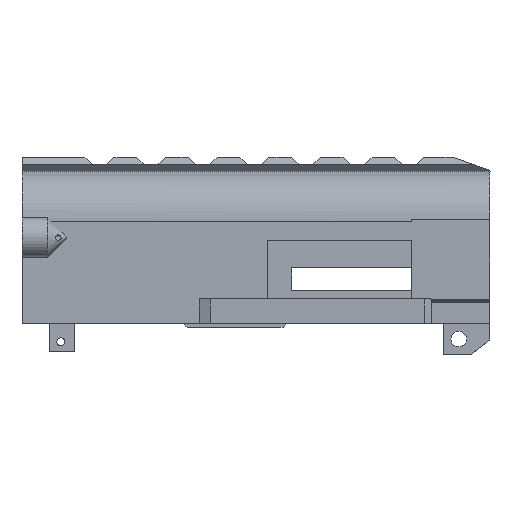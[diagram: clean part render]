
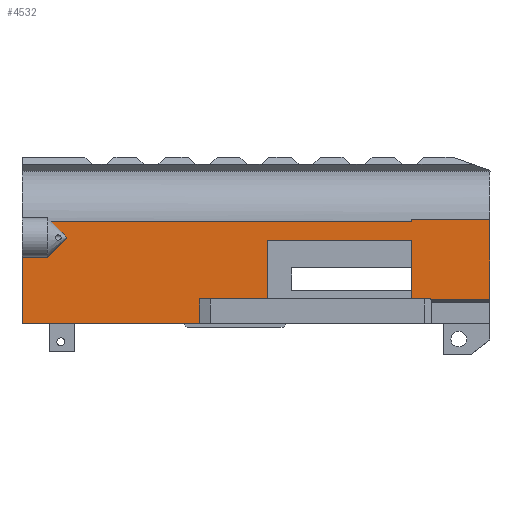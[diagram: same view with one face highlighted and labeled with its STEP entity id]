
A CAD part, top view. The second image highlights one B-rep face of the part: STEP entity #4532.
In plain terms, the highlighted planar face has unit normal (0, 0, 1).
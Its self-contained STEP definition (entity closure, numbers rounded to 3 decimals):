
#65 = CARTESIAN_POINT ( 'NONE',  ( -19.05, 16.229, 20.1 ) ) ;
#80 = VERTEX_POINT ( 'NONE', #4451 ) ;
#230 = CARTESIAN_POINT ( 'NONE',  ( -53.554, 16.363, 20.1 ) ) ;
#297 = DIRECTION ( 'NONE',  ( -1., 0., 0. ) ) ;
#432 = CARTESIAN_POINT ( 'NONE',  ( -11.605, 5.648, 20.1 ) ) ;
#480 = ORIENTED_EDGE ( 'NONE', *, *, #613, .F. ) ;
#537 = CARTESIAN_POINT ( 'NONE',  ( -167.482, 33.3, 20.1 ) ) ;
#572 = DIRECTION ( 'NONE',  ( 0.707, -0.707, 0. ) ) ;
#579 = VERTEX_POINT ( 'NONE', #3620 ) ;
#612 = LINE ( 'NONE', #2667, #9085 ) ;
#613 = EDGE_CURVE ( 'NONE', #3606, #579, #7584, .T. ) ;
#638 = DIRECTION ( 'NONE',  ( 1., 0., 0. ) ) ;
#674 = EDGE_LOOP ( 'NONE', ( #7659, #3589, #480, #2701, #2928, #7825, #6743, #4320, #2395, #4834, #3964, #5488, #8980, #8319, #5540, #8582, #5703, #3328 ) ) ;
#764 = VERTEX_POINT ( 'NONE', #1756 ) ;
#797 = EDGE_CURVE ( 'NONE', #6819, #8381, #4571, .T. ) ;
#798 = DIRECTION ( 'NONE',  ( -1., 0., 0. ) ) ;
#834 = AXIS2_PLACEMENT_3D ( 'NONE', #6555, #2433, #5251 ) ;
#867 = LINE ( 'NONE', #8546, #1990 ) ;
#907 = CARTESIAN_POINT ( 'NONE',  ( -177.682, 6.363, 20.1 ) ) ;
#932 = CARTESIAN_POINT ( 'NONE',  ( -78., 39.948, 20.1 ) ) ;
#972 = CARTESIAN_POINT ( 'NONE',  ( -159.682, 47.463, 20.1 ) ) ;
#995 = LINE ( 'NONE', #5081, #5765 ) ;
#1028 = VECTOR ( 'NONE', #638, 1000. ) ;
#1035 = DIRECTION ( 'NONE',  ( 0., -1., 0. ) ) ;
#1101 = VERTEX_POINT ( 'NONE', #8538 ) ;
#1129 = VECTOR ( 'NONE', #1190, 1000. ) ;
#1165 = LINE ( 'NONE', #7304, #7152 ) ;
#1190 = DIRECTION ( 'NONE',  ( -1., 0., 0. ) ) ;
#1319 = VERTEX_POINT ( 'NONE', #7970 ) ;
#1375 = CARTESIAN_POINT ( 'NONE',  ( -78., 16.363, 20.1 ) ) ;
#1378 = LINE ( 'NONE', #8827, #7618 ) ;
#1498 = CARTESIAN_POINT ( 'NONE',  ( -53.554, 16.363, 20.1 ) ) ;
#1505 = DIRECTION ( 'NONE',  ( 0., 1., 0. ) ) ;
#1574 = VECTOR ( 'NONE', #5190, 1000. ) ;
#1577 = DIRECTION ( 'NONE',  ( 1., 0., 0. ) ) ;
#1581 = VECTOR ( 'NONE', #1035, 1000. ) ;
#1756 = CARTESIAN_POINT ( 'NONE',  ( -11.605, 16.229, 20.1 ) ) ;
#1922 = CARTESIAN_POINT ( 'NONE',  ( -39.772, 39.948, 20.1 ) ) ;
#1963 = EDGE_CURVE ( 'NONE', #5956, #764, #5717, .T. ) ;
#1990 = VECTOR ( 'NONE', #1505, 1000. ) ;
#2395 = ORIENTED_EDGE ( 'NONE', *, *, #9096, .F. ) ;
#2433 = DIRECTION ( 'NONE',  ( 0., 0., 1. ) ) ;
#2667 = CARTESIAN_POINT ( 'NONE',  ( -159.482, 41.3, 20.1 ) ) ;
#2699 = LINE ( 'NONE', #972, #1581 ) ;
#2701 = ORIENTED_EDGE ( 'NONE', *, *, #6068, .T. ) ;
#2803 = VECTOR ( 'NONE', #6584, 1000. ) ;
#2820 = EDGE_CURVE ( 'NONE', #5543, #8736, #8386, .T. ) ;
#2871 = CARTESIAN_POINT ( 'NONE',  ( -105.565, 6.363, 20.1 ) ) ;
#2928 = ORIENTED_EDGE ( 'NONE', *, *, #7368, .F. ) ;
#3069 = CARTESIAN_POINT ( 'NONE',  ( -19.032, 39.948, 20.1 ) ) ;
#3086 = PLANE ( 'NONE',  #834 ) ;
#3224 = CARTESIAN_POINT ( 'NONE',  ( -159.682, 41.1, 20.1 ) ) ;
#3283 = LINE ( 'NONE', #4553, #7811 ) ;
#3308 = DIRECTION ( 'NONE',  ( 0., -1., 0. ) ) ;
#3311 = CARTESIAN_POINT ( 'NONE',  ( -43.5, 6.363, 20.1 ) ) ;
#3328 = ORIENTED_EDGE ( 'NONE', *, *, #6326, .T. ) ;
#3572 = LINE ( 'NONE', #4238, #7133 ) ;
#3589 = ORIENTED_EDGE ( 'NONE', *, *, #6388, .F. ) ;
#3606 = VERTEX_POINT ( 'NONE', #1375 ) ;
#3620 = CARTESIAN_POINT ( 'NONE',  ( -105.565, 16.363, 20.1 ) ) ;
#3641 = VECTOR ( 'NONE', #798, 1000. ) ;
#3696 = VECTOR ( 'NONE', #5900, 1000. ) ;
#3893 = EDGE_CURVE ( 'NONE', #7514, #8736, #2699, .T. ) ;
#3907 = VECTOR ( 'NONE', #6420, 1000. ) ;
#3964 = ORIENTED_EDGE ( 'NONE', *, *, #7773, .F. ) ;
#4229 = CARTESIAN_POINT ( 'NONE',  ( 12.7, 16.229, 20.1 ) ) ;
#4238 = CARTESIAN_POINT ( 'NONE',  ( -78., 16.363, 20.1 ) ) ;
#4274 = VERTEX_POINT ( 'NONE', #5538 ) ;
#4320 = ORIENTED_EDGE ( 'NONE', *, *, #1963, .T. ) ;
#4370 = LINE ( 'NONE', #6551, #3696 ) ;
#4398 = DIRECTION ( 'NONE',  ( 0.707, 0.707, 0. ) ) ;
#4413 = CARTESIAN_POINT ( 'NONE',  ( -11.605, 16.363, 20.1 ) ) ;
#4451 = CARTESIAN_POINT ( 'NONE',  ( 12.7, 48.532, 20.1 ) ) ;
#4532 = ADVANCED_FACE ( 'NONE', ( #6019 ), #3086, .T. ) ;
#4553 = CARTESIAN_POINT ( 'NONE',  ( -167.682, 33.3, 20.1 ) ) ;
#4571 = LINE ( 'NONE', #7162, #3907 ) ;
#4792 = EDGE_CURVE ( 'NONE', #1101, #7514, #612, .T. ) ;
#4834 = ORIENTED_EDGE ( 'NONE', *, *, #8320, .T. ) ;
#4893 = VERTEX_POINT ( 'NONE', #4229 ) ;
#4985 = LINE ( 'NONE', #1498, #3641 ) ;
#5081 = CARTESIAN_POINT ( 'NONE',  ( -19.05, 47.913, 20.1 ) ) ;
#5183 = VERTEX_POINT ( 'NONE', #907 ) ;
#5190 = DIRECTION ( 'NONE',  ( -1., 0., 0. ) ) ;
#5215 = EDGE_CURVE ( 'NONE', #5543, #4274, #3283, .T. ) ;
#5251 = DIRECTION ( 'NONE',  ( -1., 0., 0. ) ) ;
#5271 = LINE ( 'NONE', #3311, #1028 ) ;
#5286 = VECTOR ( 'NONE', #3308, 1000. ) ;
#5314 = DIRECTION ( 'NONE',  ( 0., 1., 0. ) ) ;
#5383 = LINE ( 'NONE', #5841, #2803 ) ;
#5488 = ORIENTED_EDGE ( 'NONE', *, *, #7914, .F. ) ;
#5538 = CARTESIAN_POINT ( 'NONE',  ( -177.682, 33.3, 20.1 ) ) ;
#5540 = ORIENTED_EDGE ( 'NONE', *, *, #3893, .T. ) ;
#5543 = VERTEX_POINT ( 'NONE', #537 ) ;
#5703 = ORIENTED_EDGE ( 'NONE', *, *, #5215, .T. ) ;
#5717 = LINE ( 'NONE', #432, #5286 ) ;
#5765 = VECTOR ( 'NONE', #7116, 1000. ) ;
#5841 = CARTESIAN_POINT ( 'NONE',  ( -177.682, 12.778, 20.1 ) ) ;
#5900 = DIRECTION ( 'NONE',  ( 0., -1., 0. ) ) ;
#5956 = VERTEX_POINT ( 'NONE', #4413 ) ;
#6019 = FACE_OUTER_BOUND ( 'NONE', #674, .T. ) ;
#6048 = EDGE_CURVE ( 'NONE', #5183, #8309, #5271, .T. ) ;
#6068 = EDGE_CURVE ( 'NONE', #3606, #7238, #3572, .T. ) ;
#6157 = DIRECTION ( 'NONE',  ( 0., 1., 0. ) ) ;
#6326 = EDGE_CURVE ( 'NONE', #4274, #5183, #5383, .T. ) ;
#6388 = EDGE_CURVE ( 'NONE', #579, #8309, #4370, .T. ) ;
#6420 = DIRECTION ( 'NONE',  ( 0., 1., 0. ) ) ;
#6539 = LINE ( 'NONE', #65, #7769 ) ;
#6551 = CARTESIAN_POINT ( 'NONE',  ( -105.565, 0.648, 20.1 ) ) ;
#6555 = CARTESIAN_POINT ( 'NONE',  ( -1.544, -5.067, 20.1 ) ) ;
#6584 = DIRECTION ( 'NONE',  ( 0., -1., 0. ) ) ;
#6743 = ORIENTED_EDGE ( 'NONE', *, *, #8494, .F. ) ;
#6805 = LINE ( 'NONE', #1922, #1129 ) ;
#6819 = VERTEX_POINT ( 'NONE', #7776 ) ;
#7116 = DIRECTION ( 'NONE',  ( -1., 0., 0. ) ) ;
#7133 = VECTOR ( 'NONE', #6157, 1000. ) ;
#7152 = VECTOR ( 'NONE', #1577, 1000. ) ;
#7162 = CARTESIAN_POINT ( 'NONE',  ( -19.032, 17.441, 20.1 ) ) ;
#7180 = DIRECTION ( 'NONE',  ( -1., 0., 0. ) ) ;
#7218 = CARTESIAN_POINT ( 'NONE',  ( -159.482, 41.3, 20.1 ) ) ;
#7238 = VERTEX_POINT ( 'NONE', #932 ) ;
#7304 = CARTESIAN_POINT ( 'NONE',  ( -97.797, 48.532, 20.1 ) ) ;
#7368 = EDGE_CURVE ( 'NONE', #8381, #7238, #6805, .T. ) ;
#7514 = VERTEX_POINT ( 'NONE', #7678 ) ;
#7584 = LINE ( 'NONE', #230, #1574 ) ;
#7618 = VECTOR ( 'NONE', #5314, 1000. ) ;
#7659 = ORIENTED_EDGE ( 'NONE', *, *, #6048, .T. ) ;
#7678 = CARTESIAN_POINT ( 'NONE',  ( -159.682, 41.5, 20.1 ) ) ;
#7769 = VECTOR ( 'NONE', #7180, 1000. ) ;
#7773 = EDGE_CURVE ( 'NONE', #8819, #80, #1165, .T. ) ;
#7776 = CARTESIAN_POINT ( 'NONE',  ( -19.032, 16.363, 20.1 ) ) ;
#7811 = VECTOR ( 'NONE', #297, 1000. ) ;
#7825 = ORIENTED_EDGE ( 'NONE', *, *, #797, .F. ) ;
#7914 = EDGE_CURVE ( 'NONE', #1319, #8819, #1378, .T. ) ;
#7970 = CARTESIAN_POINT ( 'NONE',  ( -19.05, 47.913, 20.1 ) ) ;
#8175 = VECTOR ( 'NONE', #4398, 1000. ) ;
#8235 = EDGE_CURVE ( 'NONE', #1319, #1101, #995, .T. ) ;
#8309 = VERTEX_POINT ( 'NONE', #2871 ) ;
#8319 = ORIENTED_EDGE ( 'NONE', *, *, #4792, .T. ) ;
#8320 = EDGE_CURVE ( 'NONE', #4893, #80, #867, .T. ) ;
#8381 = VERTEX_POINT ( 'NONE', #3069 ) ;
#8386 = LINE ( 'NONE', #7218, #8175 ) ;
#8494 = EDGE_CURVE ( 'NONE', #5956, #6819, #4985, .T. ) ;
#8538 = CARTESIAN_POINT ( 'NONE',  ( -166.095, 47.913, 20.1 ) ) ;
#8546 = CARTESIAN_POINT ( 'NONE',  ( 12.7, 4.007, 20.1 ) ) ;
#8582 = ORIENTED_EDGE ( 'NONE', *, *, #2820, .F. ) ;
#8736 = VERTEX_POINT ( 'NONE', #3224 ) ;
#8819 = VERTEX_POINT ( 'NONE', #8944 ) ;
#8827 = CARTESIAN_POINT ( 'NONE',  ( -19.05, 4.007, 20.1 ) ) ;
#8944 = CARTESIAN_POINT ( 'NONE',  ( -19.05, 48.532, 20.1 ) ) ;
#8980 = ORIENTED_EDGE ( 'NONE', *, *, #8235, .T. ) ;
#9085 = VECTOR ( 'NONE', #572, 1000. ) ;
#9096 = EDGE_CURVE ( 'NONE', #4893, #764, #6539, .T. ) ;
